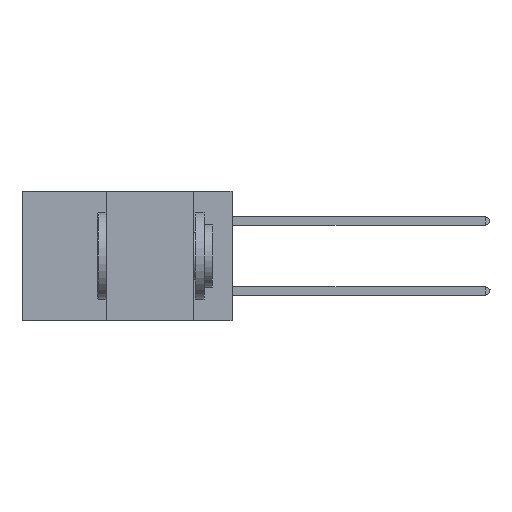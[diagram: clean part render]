
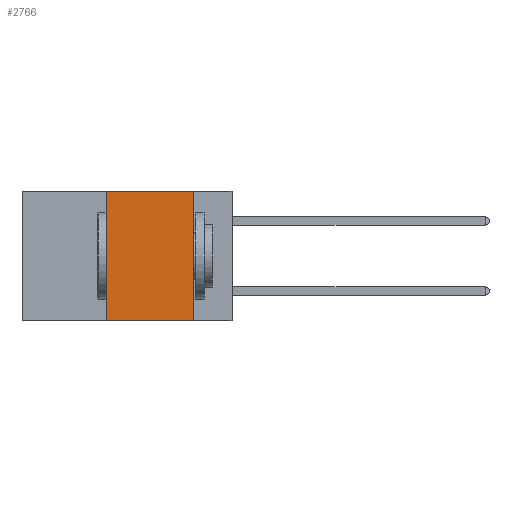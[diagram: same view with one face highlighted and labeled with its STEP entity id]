
A CAD part, left-side view. The second image highlights one B-rep face of the part: STEP entity #2766.
In plain terms, the highlighted planar face has unit normal (-1, 0, 0).
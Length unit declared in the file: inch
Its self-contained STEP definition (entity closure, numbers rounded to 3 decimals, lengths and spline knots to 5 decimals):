
#859 = ORIENTED_EDGE ( 'NONE', *, *, #3049, .T. ) ;
#1287 = DIRECTION ( 'NONE',  ( 0., 0., -1. ) ) ;
#2766 = ADVANCED_FACE ( 'NONE', ( #22035 ), #21349, .F. ) ;
#2961 = CARTESIAN_POINT ( 'NONE',  ( 0., 0.6, -0.37 ) ) ;
#3049 = EDGE_CURVE ( 'NONE', #10837, #11316, #4519, .T. ) ;
#3831 = VECTOR ( 'NONE', #21909, 39.37008 ) ;
#4519 = LINE ( 'NONE', #2961, #22923 ) ;
#5856 = CARTESIAN_POINT ( 'NONE',  ( 0., 0.11, 0. ) ) ;
#6868 = ORIENTED_EDGE ( 'NONE', *, *, #13438, .F. ) ;
#7756 = DIRECTION ( 'NONE',  ( 0., -1., 0. ) ) ;
#8245 = CARTESIAN_POINT ( 'NONE',  ( 0., 0.36, 0. ) ) ;
#8403 = VERTEX_POINT ( 'NONE', #10264 ) ;
#8663 = EDGE_CURVE ( 'NONE', #8403, #11316, #18902, .T. ) ;
#10264 = CARTESIAN_POINT ( 'NONE',  ( 0., 0.11, 0. ) ) ;
#10267 = DIRECTION ( 'NONE',  ( 0., -1., 0. ) ) ;
#10526 = CARTESIAN_POINT ( 'NONE',  ( 0., 0.6, 0. ) ) ;
#10792 = ORIENTED_EDGE ( 'NONE', *, *, #8663, .F. ) ;
#10837 = VERTEX_POINT ( 'NONE', #11240 ) ;
#10890 = VECTOR ( 'NONE', #16633, 39.37008 ) ;
#11240 = CARTESIAN_POINT ( 'NONE',  ( 0., 0.36, -0.37 ) ) ;
#11316 = VERTEX_POINT ( 'NONE', #23479 ) ;
#11346 = ORIENTED_EDGE ( 'NONE', *, *, #14643, .F. ) ;
#11649 = LINE ( 'NONE', #14919, #11925 ) ;
#11925 = VECTOR ( 'NONE', #7756, 39.37008 ) ;
#12379 = DIRECTION ( 'NONE',  ( 1., 0., 0. ) ) ;
#13075 = CARTESIAN_POINT ( 'NONE',  ( 0., 0.36, 0. ) ) ;
#13438 = EDGE_CURVE ( 'NONE', #16228, #8403, #11649, .T. ) ;
#14643 = EDGE_CURVE ( 'NONE', #10837, #16228, #15339, .T. ) ;
#14708 = AXIS2_PLACEMENT_3D ( 'NONE', #10526, #12379, #1287 ) ;
#14919 = CARTESIAN_POINT ( 'NONE',  ( 0., 0.6, 0. ) ) ;
#15339 = LINE ( 'NONE', #13075, #3831 ) ;
#16228 = VERTEX_POINT ( 'NONE', #8245 ) ;
#16633 = DIRECTION ( 'NONE',  ( 0., 0., -1. ) ) ;
#17716 = EDGE_LOOP ( 'NONE', ( #10792, #6868, #11346, #859 ) ) ;
#18902 = LINE ( 'NONE', #5856, #10890 ) ;
#21349 = PLANE ( 'NONE',  #14708 ) ;
#21909 = DIRECTION ( 'NONE',  ( 0., 0., 1. ) ) ;
#22035 = FACE_OUTER_BOUND ( 'NONE', #17716, .T. ) ;
#22923 = VECTOR ( 'NONE', #10267, 39.37008 ) ;
#23479 = CARTESIAN_POINT ( 'NONE',  ( 0., 0.11, -0.37 ) ) ;
